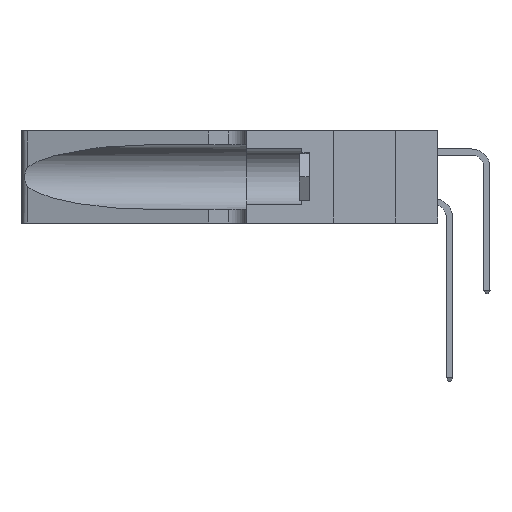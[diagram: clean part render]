
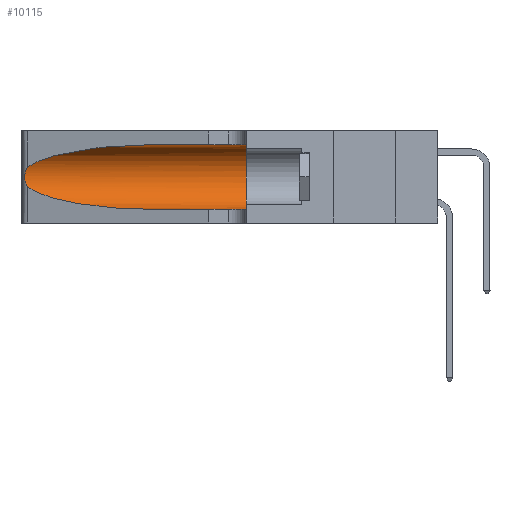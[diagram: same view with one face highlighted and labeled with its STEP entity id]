
A CAD part, left-side view. The second image highlights one B-rep face of the part: STEP entity #10115.
In plain terms, the highlighted cylindrical face has radius 3.308 mm (diameter 6.617 mm), a partial arc.
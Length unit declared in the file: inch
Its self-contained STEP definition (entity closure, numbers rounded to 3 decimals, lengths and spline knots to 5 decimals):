
#515 = CARTESIAN_POINT ( 'NONE',  ( 0.25555, 1.22994, 0.2215 ) ) ;
#757 = ORIENTED_EDGE ( 'NONE', *, *, #24057, .F. ) ;
#939 = EDGE_CURVE ( 'NONE', #15418, #25923, #2159, .T. ) ;
#1577 = VERTEX_POINT ( 'NONE', #18328 ) ;
#1692 = CARTESIAN_POINT ( 'NONE',  ( 0.1305, 1.61858, 0.05475 ) ) ;
#2159 =( BOUNDED_CURVE ( )  B_SPLINE_CURVE ( 3, ( #15170, #5066, #8419, #38553 ),
 .UNSPECIFIED., .F., .F. ) 
 B_SPLINE_CURVE_WITH_KNOTS ( ( 4, 4 ),
 ( 1.5708, 2.84003 ),
 .UNSPECIFIED. ) 
 CURVE ( )  GEOMETRIC_REPRESENTATION_ITEM ( )  RATIONAL_B_SPLINE_CURVE ( ( 1., 0.87, 0.87, 1. ) ) 
 REPRESENTATION_ITEM ( '' )  );
#2220 = VERTEX_POINT ( 'NONE', #34660 ) ;
#2406 = VECTOR ( 'NONE', #12925, 39.37008 ) ;
#3308 = DIRECTION ( 'NONE',  ( 0., 0., -1. ) ) ;
#3516 =( BOUNDED_CURVE ( )  B_SPLINE_CURVE ( 3, ( #10911, #14288, #37659, #17632 ),
 .UNSPECIFIED., .F., .F. ) 
 B_SPLINE_CURVE_WITH_KNOTS ( ( 4, 4 ),
 ( 3.44316, 4.71239 ),
 .UNSPECIFIED. ) 
 CURVE ( )  GEOMETRIC_REPRESENTATION_ITEM ( )  RATIONAL_B_SPLINE_CURVE ( ( 1., 0.87, 0.87, 1. ) ) 
 REPRESENTATION_ITEM ( '' )  );
#3703 = DIRECTION ( 'NONE',  ( 0., 1., 0. ) ) ;
#3974 = CARTESIAN_POINT ( 'NONE',  ( 0.25787, 1.23484, 0.2124 ) ) ;
#5066 = CARTESIAN_POINT ( 'NONE',  ( 0.18966, 0.96281, 0.31525 ) ) ;
#5467 = CARTESIAN_POINT ( 'NONE',  ( 0.1305, 0.72297, 0.31525 ) ) ;
#7355 = CARTESIAN_POINT ( 'NONE',  ( 0.26018, 1.23835, 0.19895 ) ) ;
#8419 = CARTESIAN_POINT ( 'NONE',  ( 0.2373, 1.15595, 0.28018 ) ) ;
#8503 = LINE ( 'NONE', #1692, #34156 ) ;
#9567 = CARTESIAN_POINT ( 'NONE',  ( 0.1305, 1.61858, 0.31525 ) ) ;
#10115 = ADVANCED_FACE ( 'NONE', ( #18242 ), #17172, .F. ) ;
#10131 = AXIS2_PLACEMENT_3D ( 'NONE', #40086, #23386, #3308 ) ;
#10722 = CARTESIAN_POINT ( 'NONE',  ( 0.26075, 1.23896, 0.178 ) ) ;
#10877 = ORIENTED_EDGE ( 'NONE', *, *, #41182, .T. ) ;
#10911 = CARTESIAN_POINT ( 'NONE',  ( 0.25487, 1.22718, 0.14631 ) ) ;
#12814 = EDGE_CURVE ( 'NONE', #25923, #43170, #42417, .T. ) ;
#12925 = DIRECTION ( 'NONE',  ( 0., -1., 0. ) ) ;
#14093 = CARTESIAN_POINT ( 'NONE',  ( 0.25856, 1.23593, 0.16098 ) ) ;
#14288 = CARTESIAN_POINT ( 'NONE',  ( 0.2373, 1.15595, 0.08982 ) ) ;
#15117 = ORIENTED_EDGE ( 'NONE', *, *, #12814, .T. ) ;
#15170 = CARTESIAN_POINT ( 'NONE',  ( 0.1305, 0.72297, 0.31525 ) ) ;
#15225 = ORIENTED_EDGE ( 'NONE', *, *, #24176, .T. ) ;
#15418 = VERTEX_POINT ( 'NONE', #5467 ) ;
#17172 = CYLINDRICAL_SURFACE ( 'NONE', #10131, 0.13025 ) ;
#17437 = CARTESIAN_POINT ( 'NONE',  ( 0.25639, 1.23186, 0.15144 ) ) ;
#17632 = CARTESIAN_POINT ( 'NONE',  ( 0.1305, 0.72297, 0.05475 ) ) ;
#18100 = CARTESIAN_POINT ( 'NONE',  ( 0.25487, 1.22718, 0.14631 ) ) ;
#18242 = FACE_OUTER_BOUND ( 'NONE', #35948, .T. ) ;
#18328 = CARTESIAN_POINT ( 'NONE',  ( 0.1305, 0.35, 0.05475 ) ) ;
#20279 = LINE ( 'NONE', #9567, #2406 ) ;
#20814 = CARTESIAN_POINT ( 'NONE',  ( 0.25487, 1.22718, 0.14631 ) ) ;
#20966 = CARTESIAN_POINT ( 'NONE',  ( 0.1305, 0.72297, 0.05475 ) ) ;
#21812 = DIRECTION ( 'NONE',  ( 0., -1., 0. ) ) ;
#23386 = DIRECTION ( 'NONE',  ( 0., -1., 0. ) ) ;
#23775 = CARTESIAN_POINT ( 'NONE',  ( 0.1305, 0.35, 0.185 ) ) ;
#24041 = CARTESIAN_POINT ( 'NONE',  ( 0.25639, 1.23184, 0.21858 ) ) ;
#24057 = EDGE_CURVE ( 'NONE', #2220, #1577, #28204, .T. ) ;
#24176 = EDGE_CURVE ( 'NONE', #43170, #36998, #3516, .T. ) ;
#24912 = EDGE_CURVE ( 'NONE', #15418, #2220, #20279, .T. ) ;
#25169 = AXIS2_PLACEMENT_3D ( 'NONE', #23775, #3703, #27148 ) ;
#25923 = VERTEX_POINT ( 'NONE', #28228 ) ;
#27148 = DIRECTION ( 'NONE',  ( 0., 0., 1. ) ) ;
#27393 = CARTESIAN_POINT ( 'NONE',  ( 0.25854, 1.2359, 0.20912 ) ) ;
#28204 = CIRCLE ( 'NONE', #25169, 0.13025 ) ;
#28228 = CARTESIAN_POINT ( 'NONE',  ( 0.25487, 1.22718, 0.22369 ) ) ;
#30761 = CARTESIAN_POINT ( 'NONE',  ( 0.26075, 1.23896, 0.19203 ) ) ;
#34127 = CARTESIAN_POINT ( 'NONE',  ( 0.26017, 1.23833, 0.17102 ) ) ;
#34156 = VECTOR ( 'NONE', #21812, 39.37008 ) ;
#34261 = ORIENTED_EDGE ( 'NONE', *, *, #24912, .F. ) ;
#34660 = CARTESIAN_POINT ( 'NONE',  ( 0.1305, 0.35, 0.31525 ) ) ;
#35948 = EDGE_LOOP ( 'NONE', ( #40168, #15117, #15225, #10877, #757, #34261 ) ) ;
#36998 = VERTEX_POINT ( 'NONE', #20966 ) ;
#37479 = CARTESIAN_POINT ( 'NONE',  ( 0.25789, 1.23486, 0.15765 ) ) ;
#37659 = CARTESIAN_POINT ( 'NONE',  ( 0.18966, 0.96281, 0.05475 ) ) ;
#38553 = CARTESIAN_POINT ( 'NONE',  ( 0.25487, 1.22718, 0.22369 ) ) ;
#40086 = CARTESIAN_POINT ( 'NONE',  ( 0.1305, 1.61858, 0.185 ) ) ;
#40168 = ORIENTED_EDGE ( 'NONE', *, *, #939, .T. ) ;
#40686 = CARTESIAN_POINT ( 'NONE',  ( 0.25487, 1.22718, 0.22369 ) ) ;
#40837 = CARTESIAN_POINT ( 'NONE',  ( 0.25555, 1.22993, 0.14849 ) ) ;
#41182 = EDGE_CURVE ( 'NONE', #36998, #1577, #8503, .T. ) ;
#42417 = B_SPLINE_CURVE_WITH_KNOTS ( 'NONE', 3,
 ( #40686, #515, #24041, #3974, #27393, #7355, #30761, #10722, #34127, #14093, #37479, #17437, #40837, #20814 ),
 .UNSPECIFIED., .F., .F.,
 ( 4, 2, 2, 2, 2, 2, 4 ),
 ( 0., 0.00027, 0.00053, 0.00107, 0.0016, 0.00187, 0.00214 ),
 .UNSPECIFIED. ) ;
#43170 = VERTEX_POINT ( 'NONE', #18100 ) ;
